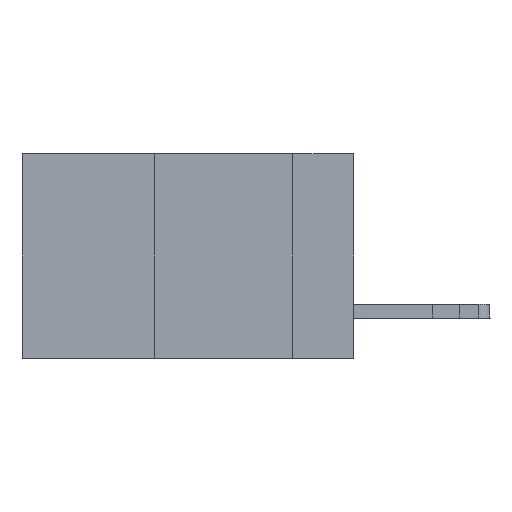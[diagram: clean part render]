
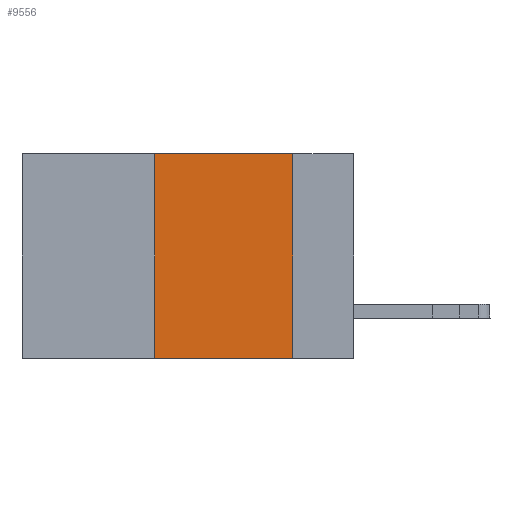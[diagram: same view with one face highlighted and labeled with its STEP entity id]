
A CAD part, left-side view. The second image highlights one B-rep face of the part: STEP entity #9556.
In plain terms, the highlighted planar face has unit normal (-1, 0, 0).
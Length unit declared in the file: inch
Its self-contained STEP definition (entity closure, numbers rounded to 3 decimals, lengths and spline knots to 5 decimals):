
#385 = DIRECTION ( 'NONE',  ( 0., -1., 0. ) ) ;
#398 = VERTEX_POINT ( 'NONE', #3439 ) ;
#1135 = EDGE_CURVE ( 'NONE', #19978, #398, #19022, .T. ) ;
#3439 = CARTESIAN_POINT ( 'NONE',  ( 0., 0.11, 0. ) ) ;
#3736 = VECTOR ( 'NONE', #8447, 39.37008 ) ;
#4075 = VECTOR ( 'NONE', #17402, 39.37008 ) ;
#4489 = AXIS2_PLACEMENT_3D ( 'NONE', #17805, #7284, #19552 ) ;
#4526 = VERTEX_POINT ( 'NONE', #5644 ) ;
#5034 = CARTESIAN_POINT ( 'NONE',  ( 0., 0.36, 0. ) ) ;
#5336 = CARTESIAN_POINT ( 'NONE',  ( 0., 0.11, -0.37 ) ) ;
#5511 = CARTESIAN_POINT ( 'NONE',  ( 0., 0.36, 0. ) ) ;
#5644 = CARTESIAN_POINT ( 'NONE',  ( 0., 0.36, -0.37 ) ) ;
#6258 = ORIENTED_EDGE ( 'NONE', *, *, #17933, .F. ) ;
#7284 = DIRECTION ( 'NONE',  ( 1., 0., 0. ) ) ;
#8447 = DIRECTION ( 'NONE',  ( 0., 0., -1. ) ) ;
#9071 = LINE ( 'NONE', #22395, #3736 ) ;
#9122 = FACE_OUTER_BOUND ( 'NONE', #22173, .T. ) ;
#9450 = CARTESIAN_POINT ( 'NONE',  ( 0., 0.6, -0.37 ) ) ;
#9556 = ADVANCED_FACE ( 'NONE', ( #9122 ), #12401, .F. ) ;
#9711 = EDGE_CURVE ( 'NONE', #4526, #10638, #19792, .T. ) ;
#10511 = VECTOR ( 'NONE', #385, 39.37008 ) ;
#10638 = VERTEX_POINT ( 'NONE', #5336 ) ;
#12401 = PLANE ( 'NONE',  #4489 ) ;
#13339 = CARTESIAN_POINT ( 'NONE',  ( 0., 0.6, 0. ) ) ;
#14369 = VECTOR ( 'NONE', #20669, 39.37008 ) ;
#16593 = ORIENTED_EDGE ( 'NONE', *, *, #19066, .F. ) ;
#16713 = ORIENTED_EDGE ( 'NONE', *, *, #1135, .F. ) ;
#17402 = DIRECTION ( 'NONE',  ( 0., 0., 1. ) ) ;
#17634 = LINE ( 'NONE', #5034, #4075 ) ;
#17805 = CARTESIAN_POINT ( 'NONE',  ( 0., 0.6, 0. ) ) ;
#17933 = EDGE_CURVE ( 'NONE', #4526, #19978, #17634, .T. ) ;
#19022 = LINE ( 'NONE', #13339, #14369 ) ;
#19066 = EDGE_CURVE ( 'NONE', #398, #10638, #9071, .T. ) ;
#19552 = DIRECTION ( 'NONE',  ( 0., 0., -1. ) ) ;
#19792 = LINE ( 'NONE', #9450, #10511 ) ;
#19978 = VERTEX_POINT ( 'NONE', #5511 ) ;
#20669 = DIRECTION ( 'NONE',  ( 0., -1., 0. ) ) ;
#22173 = EDGE_LOOP ( 'NONE', ( #16593, #16713, #6258, #22621 ) ) ;
#22395 = CARTESIAN_POINT ( 'NONE',  ( 0., 0.11, 0. ) ) ;
#22621 = ORIENTED_EDGE ( 'NONE', *, *, #9711, .T. ) ;
